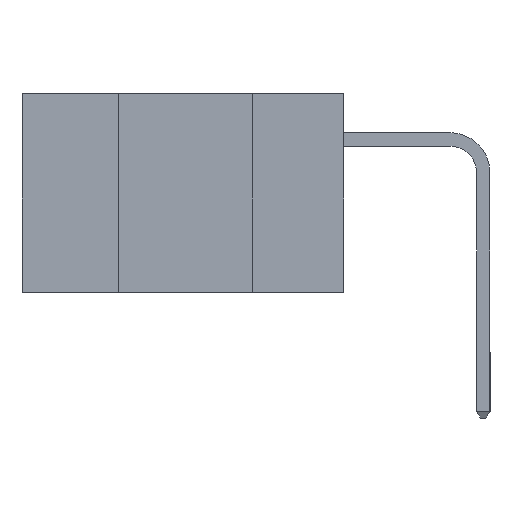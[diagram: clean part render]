
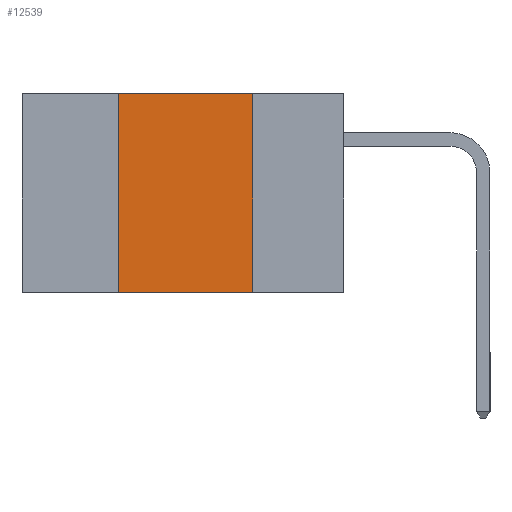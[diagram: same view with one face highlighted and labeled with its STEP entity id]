
A CAD part, left-side view. The second image highlights one B-rep face of the part: STEP entity #12539.
In plain terms, the highlighted planar face has unit normal (-1, 0, 0).
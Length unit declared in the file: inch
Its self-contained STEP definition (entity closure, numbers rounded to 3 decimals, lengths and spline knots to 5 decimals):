
#165 = FACE_OUTER_BOUND ( 'NONE', #8950, .T. ) ;
#469 = LINE ( 'NONE', #5037, #8750 ) ;
#749 = VERTEX_POINT ( 'NONE', #11640 ) ;
#871 = LINE ( 'NONE', #7912, #7629 ) ;
#1120 = LINE ( 'NONE', #12492, #3044 ) ;
#2400 = DIRECTION ( 'NONE',  ( 0., -1., 0. ) ) ;
#2419 = EDGE_CURVE ( 'NONE', #14136, #14307, #469, .T. ) ;
#3044 = VECTOR ( 'NONE', #6798, 39.37008 ) ;
#4304 = ORIENTED_EDGE ( 'NONE', *, *, #2419, .F. ) ;
#4434 = DIRECTION ( 'NONE',  ( 0., 0., -1. ) ) ;
#4498 = VECTOR ( 'NONE', #2400, 39.37008 ) ;
#5037 = CARTESIAN_POINT ( 'NONE',  ( 0., 0.42, -0.37 ) ) ;
#5783 = EDGE_CURVE ( 'NONE', #14307, #749, #1120, .T. ) ;
#6007 = CARTESIAN_POINT ( 'NONE',  ( 0., 0.42, 0. ) ) ;
#6638 = DIRECTION ( 'NONE',  ( 0., 0., -1. ) ) ;
#6798 = DIRECTION ( 'NONE',  ( 0., -1., 0. ) ) ;
#6995 = AXIS2_PLACEMENT_3D ( 'NONE', #11327, #14718, #4434 ) ;
#7629 = VECTOR ( 'NONE', #6638, 39.37008 ) ;
#7912 = CARTESIAN_POINT ( 'NONE',  ( 0., 0.17, -0.37 ) ) ;
#8117 = CARTESIAN_POINT ( 'NONE',  ( 0., 0.6, -0.37 ) ) ;
#8750 = VECTOR ( 'NONE', #14011, 39.37008 ) ;
#8950 = EDGE_LOOP ( 'NONE', ( #11890, #9262, #4304, #12571 ) ) ;
#9175 = CARTESIAN_POINT ( 'NONE',  ( 0., 0.17, -0.37 ) ) ;
#9262 = ORIENTED_EDGE ( 'NONE', *, *, #5783, .F. ) ;
#11327 = CARTESIAN_POINT ( 'NONE',  ( 0., 0.6, 0. ) ) ;
#11477 = LINE ( 'NONE', #8117, #4498 ) ;
#11640 = CARTESIAN_POINT ( 'NONE',  ( 0., 0.17, 0. ) ) ;
#11890 = ORIENTED_EDGE ( 'NONE', *, *, #13268, .F. ) ;
#12346 = CARTESIAN_POINT ( 'NONE',  ( 0., 0.42, -0.37 ) ) ;
#12458 = PLANE ( 'NONE',  #6995 ) ;
#12492 = CARTESIAN_POINT ( 'NONE',  ( 0., 0.6, 0. ) ) ;
#12539 = ADVANCED_FACE ( 'NONE', ( #165 ), #12458, .F. ) ;
#12571 = ORIENTED_EDGE ( 'NONE', *, *, #13912, .T. ) ;
#13268 = EDGE_CURVE ( 'NONE', #749, #14778, #871, .T. ) ;
#13912 = EDGE_CURVE ( 'NONE', #14136, #14778, #11477, .T. ) ;
#14011 = DIRECTION ( 'NONE',  ( 0., 0., 1. ) ) ;
#14136 = VERTEX_POINT ( 'NONE', #12346 ) ;
#14307 = VERTEX_POINT ( 'NONE', #6007 ) ;
#14718 = DIRECTION ( 'NONE',  ( 1., 0., 0. ) ) ;
#14778 = VERTEX_POINT ( 'NONE', #9175 ) ;
